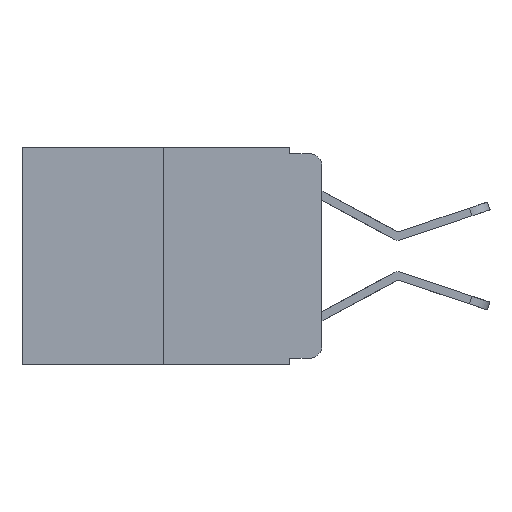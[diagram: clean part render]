
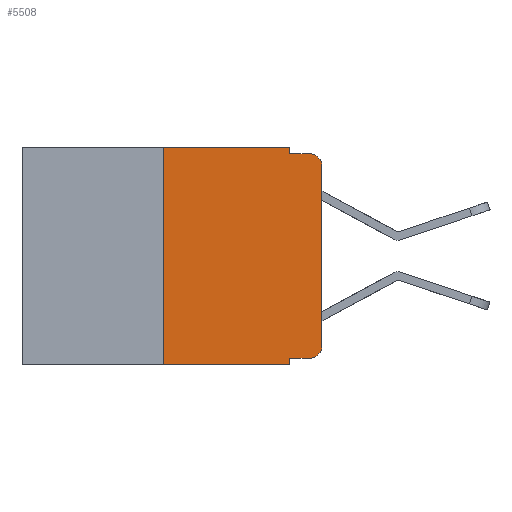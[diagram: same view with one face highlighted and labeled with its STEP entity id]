
A CAD part, left-side view. The second image highlights one B-rep face of the part: STEP entity #5508.
In plain terms, the highlighted planar face has unit normal (-1, 0, 0).
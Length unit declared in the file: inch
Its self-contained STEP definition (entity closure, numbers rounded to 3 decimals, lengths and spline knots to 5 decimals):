
#187 = DIRECTION ( 'NONE',  ( 0., -1., 0. ) ) ;
#653 = PLANE ( 'NONE',  #4684 ) ;
#983 = VERTEX_POINT ( 'NONE', #26615 ) ;
#1168 = DIRECTION ( 'NONE',  ( 0., 0., 1. ) ) ;
#1526 = DIRECTION ( 'NONE',  ( 0., 0., -1. ) ) ;
#2078 = EDGE_CURVE ( 'NONE', #19731, #6896, #4184, .T. ) ;
#2093 = CARTESIAN_POINT ( 'NONE',  ( 0., 0.25, 0. ) ) ;
#2101 = CIRCLE ( 'NONE', #22097, 0.02 ) ;
#2596 = CARTESIAN_POINT ( 'NONE',  ( 0., 0., -0.313 ) ) ;
#2705 = LINE ( 'NONE', #17965, #18729 ) ;
#2862 = CARTESIAN_POINT ( 'NONE',  ( 0., 0.473, 0. ) ) ;
#3512 = EDGE_CURVE ( 'NONE', #15708, #20831, #2101, .T. ) ;
#4184 = LINE ( 'NONE', #13846, #8563 ) ;
#4233 = ORIENTED_EDGE ( 'NONE', *, *, #4966, .T. ) ;
#4291 = ORIENTED_EDGE ( 'NONE', *, *, #3512, .T. ) ;
#4371 = CARTESIAN_POINT ( 'NONE',  ( 0., 0.051, -0.333 ) ) ;
#4675 = ORIENTED_EDGE ( 'NONE', *, *, #26061, .F. ) ;
#4684 = AXIS2_PLACEMENT_3D ( 'NONE', #2862, #17500, #5062 ) ;
#4739 = ORIENTED_EDGE ( 'NONE', *, *, #24729, .F. ) ;
#4791 = ORIENTED_EDGE ( 'NONE', *, *, #26790, .F. ) ;
#4920 = ORIENTED_EDGE ( 'NONE', *, *, #23394, .F. ) ;
#4966 = EDGE_CURVE ( 'NONE', #15529, #15708, #2705, .T. ) ;
#5062 = DIRECTION ( 'NONE',  ( 0., 0., -1. ) ) ;
#5096 = ORIENTED_EDGE ( 'NONE', *, *, #2078, .T. ) ;
#5199 = ORIENTED_EDGE ( 'NONE', *, *, #22046, .F. ) ;
#5480 = ORIENTED_EDGE ( 'NONE', *, *, #16644, .T. ) ;
#5508 = ADVANCED_FACE ( 'NONE', ( #5747 ), #653, .F. ) ;
#5746 = ORIENTED_EDGE ( 'NONE', *, *, #13974, .T. ) ;
#5747 = FACE_OUTER_BOUND ( 'NONE', #5756, .T. ) ;
#5756 = EDGE_LOOP ( 'NONE', ( #4233, #4291, #4675, #4739, #4791, #4920, #5096, #5199, #5480, #5746 ) ) ;
#6896 = VERTEX_POINT ( 'NONE', #20382 ) ;
#6959 = VERTEX_POINT ( 'NONE', #12467 ) ;
#7366 = DIRECTION ( 'NONE',  ( 0., 0., 1. ) ) ;
#8563 = VECTOR ( 'NONE', #19936, 39.37008 ) ;
#10133 = CARTESIAN_POINT ( 'NONE',  ( 0., 0.051, 0. ) ) ;
#10297 = DIRECTION ( 'NONE',  ( 0., 0., -1. ) ) ;
#10647 = DIRECTION ( 'NONE',  ( 0., -1., 0. ) ) ;
#11501 = VECTOR ( 'NONE', #187, 39.37008 ) ;
#11661 = CARTESIAN_POINT ( 'NONE',  ( 0., 0.25, 0. ) ) ;
#11694 = CARTESIAN_POINT ( 'NONE',  ( 0., 0.02, -0.03 ) ) ;
#11747 = LINE ( 'NONE', #4371, #26507 ) ;
#12357 = DIRECTION ( 'NONE',  ( -1., 0., 0. ) ) ;
#12467 = CARTESIAN_POINT ( 'NONE',  ( 0., 0.051, -0.01 ) ) ;
#13733 = DIRECTION ( 'NONE',  ( 0., 0., -1. ) ) ;
#13846 = CARTESIAN_POINT ( 'NONE',  ( 0., 0.473, -0.343 ) ) ;
#13974 = EDGE_CURVE ( 'NONE', #18925, #15529, #24598, .T. ) ;
#14806 = VECTOR ( 'NONE', #7366, 39.37008 ) ;
#15285 = CARTESIAN_POINT ( 'NONE',  ( 0., 0.051, -0.333 ) ) ;
#15361 = DIRECTION ( 'NONE',  ( 0., -1., 0. ) ) ;
#15526 = LINE ( 'NONE', #10133, #25561 ) ;
#15529 = VERTEX_POINT ( 'NONE', #2596 ) ;
#15662 = CARTESIAN_POINT ( 'NONE',  ( 0., 0.25, -0.343 ) ) ;
#15708 = VERTEX_POINT ( 'NONE', #17874 ) ;
#16644 = EDGE_CURVE ( 'NONE', #20529, #18925, #11747, .T. ) ;
#17500 = DIRECTION ( 'NONE',  ( 1., 0., 0. ) ) ;
#17874 = CARTESIAN_POINT ( 'NONE',  ( 0., 0., -0.03 ) ) ;
#17965 = CARTESIAN_POINT ( 'NONE',  ( 0., 0., 0. ) ) ;
#18280 = CARTESIAN_POINT ( 'NONE',  ( 0., 0.02, -0.01 ) ) ;
#18391 = CARTESIAN_POINT ( 'NONE',  ( 0., 0.051, 0. ) ) ;
#18729 = VECTOR ( 'NONE', #1168, 39.37008 ) ;
#18925 = VERTEX_POINT ( 'NONE', #21229 ) ;
#19337 = CARTESIAN_POINT ( 'NONE',  ( 0., 0.473, 0. ) ) ;
#19731 = VERTEX_POINT ( 'NONE', #15662 ) ;
#19914 = AXIS2_PLACEMENT_3D ( 'NONE', #24393, #12357, #26393 ) ;
#19936 = DIRECTION ( 'NONE',  ( 0., -1., 0. ) ) ;
#20106 = VECTOR ( 'NONE', #10297, 39.37008 ) ;
#20170 = LINE ( 'NONE', #11661, #14806 ) ;
#20382 = CARTESIAN_POINT ( 'NONE',  ( 0., 0.051, -0.343 ) ) ;
#20529 = VERTEX_POINT ( 'NONE', #15285 ) ;
#20831 = VERTEX_POINT ( 'NONE', #18280 ) ;
#21229 = CARTESIAN_POINT ( 'NONE',  ( 0., 0.02, -0.333 ) ) ;
#22046 = EDGE_CURVE ( 'NONE', #20529, #6896, #15526, .T. ) ;
#22097 = AXIS2_PLACEMENT_3D ( 'NONE', #11694, #25738, #13733 ) ;
#22194 = LINE ( 'NONE', #25058, #11501 ) ;
#22198 = VERTEX_POINT ( 'NONE', #2093 ) ;
#23394 = EDGE_CURVE ( 'NONE', #19731, #22198, #20170, .T. ) ;
#24393 = CARTESIAN_POINT ( 'NONE',  ( 0., 0.02, -0.313 ) ) ;
#24598 = CIRCLE ( 'NONE', #19914, 0.02 ) ;
#24729 = EDGE_CURVE ( 'NONE', #983, #6959, #25408, .T. ) ;
#25058 = CARTESIAN_POINT ( 'NONE',  ( 0., 0.051, -0.01 ) ) ;
#25408 = LINE ( 'NONE', #18391, #20106 ) ;
#25561 = VECTOR ( 'NONE', #1526, 39.37008 ) ;
#25738 = DIRECTION ( 'NONE',  ( -1., 0., 0. ) ) ;
#25913 = VECTOR ( 'NONE', #15361, 39.37008 ) ;
#26061 = EDGE_CURVE ( 'NONE', #6959, #20831, #22194, .T. ) ;
#26393 = DIRECTION ( 'NONE',  ( 0., 0., -1. ) ) ;
#26507 = VECTOR ( 'NONE', #10647, 39.37008 ) ;
#26540 = LINE ( 'NONE', #19337, #25913 ) ;
#26615 = CARTESIAN_POINT ( 'NONE',  ( 0., 0.051, 0. ) ) ;
#26790 = EDGE_CURVE ( 'NONE', #22198, #983, #26540, .T. ) ;
